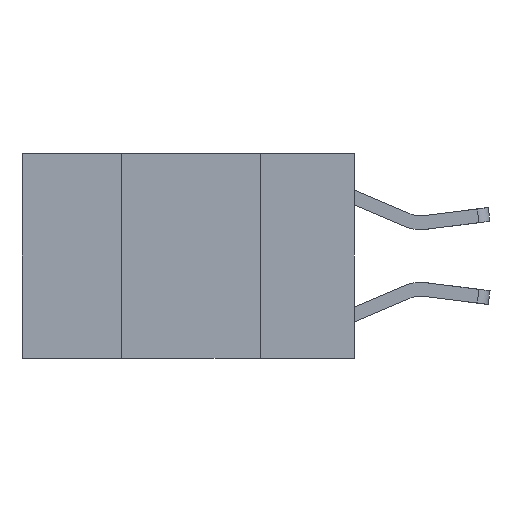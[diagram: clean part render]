
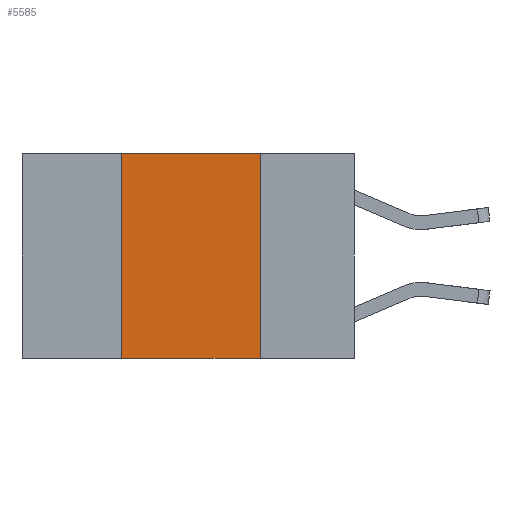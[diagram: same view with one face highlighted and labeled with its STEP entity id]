
A CAD part, left-side view. The second image highlights one B-rep face of the part: STEP entity #5585.
In plain terms, the highlighted planar face has unit normal (-1, 0, 0).
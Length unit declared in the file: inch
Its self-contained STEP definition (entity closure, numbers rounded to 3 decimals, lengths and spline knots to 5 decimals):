
#213 = CARTESIAN_POINT ( 'NONE',  ( 0., 0.17, 0. ) ) ;
#322 = ORIENTED_EDGE ( 'NONE', *, *, #470, .F. ) ;
#470 = EDGE_CURVE ( 'NONE', #9859, #2871, #9108, .T. ) ;
#563 = EDGE_CURVE ( 'NONE', #2871, #4743, #8108, .T. ) ;
#1299 = VECTOR ( 'NONE', #9040, 39.37008 ) ;
#1367 = PLANE ( 'NONE',  #7674 ) ;
#1946 = CARTESIAN_POINT ( 'NONE',  ( 0., 0.42, -0.37 ) ) ;
#2139 = ORIENTED_EDGE ( 'NONE', *, *, #7195, .F. ) ;
#2400 = CARTESIAN_POINT ( 'NONE',  ( 0., 0.17, 0. ) ) ;
#2871 = VERTEX_POINT ( 'NONE', #2400 ) ;
#3464 = LINE ( 'NONE', #8249, #1299 ) ;
#3809 = DIRECTION ( 'NONE',  ( 0., -1., 0. ) ) ;
#3814 = CARTESIAN_POINT ( 'NONE',  ( 0., 0.6, 0. ) ) ;
#4227 = CARTESIAN_POINT ( 'NONE',  ( 0., 0.42, 0. ) ) ;
#4264 = VERTEX_POINT ( 'NONE', #1946 ) ;
#4320 = DIRECTION ( 'NONE',  ( 0., -1., 0. ) ) ;
#4339 = CARTESIAN_POINT ( 'NONE',  ( 0., 0.17, -0.37 ) ) ;
#4600 = DIRECTION ( 'NONE',  ( 1., 0., 0. ) ) ;
#4743 = VERTEX_POINT ( 'NONE', #4339 ) ;
#5585 = ADVANCED_FACE ( 'NONE', ( #7897 ), #1367, .F. ) ;
#6034 = VECTOR ( 'NONE', #6935, 39.37008 ) ;
#6528 = ORIENTED_EDGE ( 'NONE', *, *, #563, .F. ) ;
#6935 = DIRECTION ( 'NONE',  ( 0., 0., -1. ) ) ;
#7023 = VECTOR ( 'NONE', #4320, 39.37008 ) ;
#7195 = EDGE_CURVE ( 'NONE', #4264, #9859, #3464, .T. ) ;
#7674 = AXIS2_PLACEMENT_3D ( 'NONE', #3814, #4600, #10077 ) ;
#7897 = FACE_OUTER_BOUND ( 'NONE', #8638, .T. ) ;
#8108 = LINE ( 'NONE', #213, #6034 ) ;
#8240 = LINE ( 'NONE', #8506, #10062 ) ;
#8249 = CARTESIAN_POINT ( 'NONE',  ( 0., 0.42, 0. ) ) ;
#8293 = EDGE_CURVE ( 'NONE', #4264, #4743, #8240, .T. ) ;
#8506 = CARTESIAN_POINT ( 'NONE',  ( 0., 0.6, -0.37 ) ) ;
#8638 = EDGE_LOOP ( 'NONE', ( #6528, #322, #2139, #8810 ) ) ;
#8810 = ORIENTED_EDGE ( 'NONE', *, *, #8293, .T. ) ;
#9040 = DIRECTION ( 'NONE',  ( 0., 0., 1. ) ) ;
#9086 = CARTESIAN_POINT ( 'NONE',  ( 0., 0.6, 0. ) ) ;
#9108 = LINE ( 'NONE', #9086, #7023 ) ;
#9859 = VERTEX_POINT ( 'NONE', #4227 ) ;
#10062 = VECTOR ( 'NONE', #3809, 39.37008 ) ;
#10077 = DIRECTION ( 'NONE',  ( 0., 0., -1. ) ) ;
